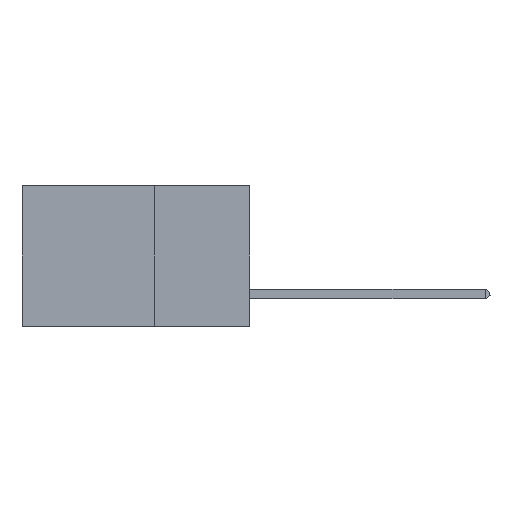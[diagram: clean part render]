
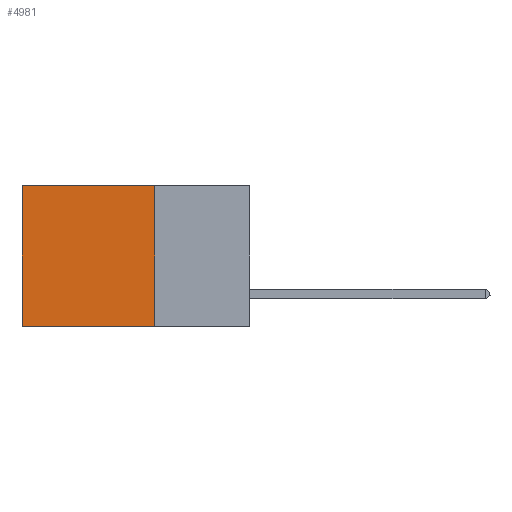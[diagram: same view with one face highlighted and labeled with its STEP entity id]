
A CAD part, left-side view. The second image highlights one B-rep face of the part: STEP entity #4981.
In plain terms, the highlighted planar face has unit normal (-1, 0, 0).
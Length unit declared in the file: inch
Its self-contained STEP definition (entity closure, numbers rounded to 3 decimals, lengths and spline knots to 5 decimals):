
#352 = VERTEX_POINT ( 'NONE', #19878 ) ;
#1156 = PLANE ( 'NONE',  #3548 ) ;
#1314 = CARTESIAN_POINT ( 'NONE',  ( 0.2875, 0.25, 0. ) ) ;
#2040 = LINE ( 'NONE', #18905, #5861 ) ;
#2269 = EDGE_CURVE ( 'NONE', #7128, #10861, #2040, .T. ) ;
#2306 = LINE ( 'NONE', #12240, #18413 ) ;
#2544 = VERTEX_POINT ( 'NONE', #16225 ) ;
#2773 = ORIENTED_EDGE ( 'NONE', *, *, #7151, .T. ) ;
#3205 = ORIENTED_EDGE ( 'NONE', *, *, #20852, .T. ) ;
#3548 = AXIS2_PLACEMENT_3D ( 'NONE', #1314, #8405, #11698 ) ;
#4609 = FACE_OUTER_BOUND ( 'NONE', #11323, .T. ) ;
#4981 = ADVANCED_FACE ( 'NONE', ( #4609 ), #1156, .F. ) ;
#5213 = ORIENTED_EDGE ( 'NONE', *, *, #2269, .F. ) ;
#5861 = VECTOR ( 'NONE', #20729, 39.37008 ) ;
#6294 = EDGE_CURVE ( 'NONE', #2544, #7128, #19025, .T. ) ;
#7116 = DIRECTION ( 'NONE',  ( 0., 0., -1. ) ) ;
#7128 = VERTEX_POINT ( 'NONE', #19924 ) ;
#7151 = EDGE_CURVE ( 'NONE', #352, #10861, #10632, .T. ) ;
#8405 = DIRECTION ( 'NONE',  ( 1., 0., 0. ) ) ;
#8857 = VECTOR ( 'NONE', #7116, 39.37008 ) ;
#10632 = LINE ( 'NONE', #19990, #12474 ) ;
#10861 = VERTEX_POINT ( 'NONE', #19105 ) ;
#11323 = EDGE_LOOP ( 'NONE', ( #2773, #5213, #21032, #3205 ) ) ;
#11698 = DIRECTION ( 'NONE',  ( 0., 0., -1. ) ) ;
#12015 = CARTESIAN_POINT ( 'NONE',  ( 0.2875, 0.25, 0. ) ) ;
#12240 = CARTESIAN_POINT ( 'NONE',  ( 0.2875, 0.25, 0. ) ) ;
#12474 = VECTOR ( 'NONE', #21697, 39.37008 ) ;
#16225 = CARTESIAN_POINT ( 'NONE',  ( 0.2875, 0.25, 0. ) ) ;
#17333 = DIRECTION ( 'NONE',  ( 0., 1., 0. ) ) ;
#18413 = VECTOR ( 'NONE', #17333, 39.37008 ) ;
#18905 = CARTESIAN_POINT ( 'NONE',  ( 0.2875, 0.25, -0.37 ) ) ;
#19025 = LINE ( 'NONE', #12015, #8857 ) ;
#19105 = CARTESIAN_POINT ( 'NONE',  ( 0.2875, 0.6, -0.37 ) ) ;
#19878 = CARTESIAN_POINT ( 'NONE',  ( 0.2875, 0.6, 0. ) ) ;
#19924 = CARTESIAN_POINT ( 'NONE',  ( 0.2875, 0.25, -0.37 ) ) ;
#19990 = CARTESIAN_POINT ( 'NONE',  ( 0.2875, 0.6, 0. ) ) ;
#20729 = DIRECTION ( 'NONE',  ( 0., 1., 0. ) ) ;
#20852 = EDGE_CURVE ( 'NONE', #2544, #352, #2306, .T. ) ;
#21032 = ORIENTED_EDGE ( 'NONE', *, *, #6294, .F. ) ;
#21697 = DIRECTION ( 'NONE',  ( 0., 0., -1. ) ) ;
